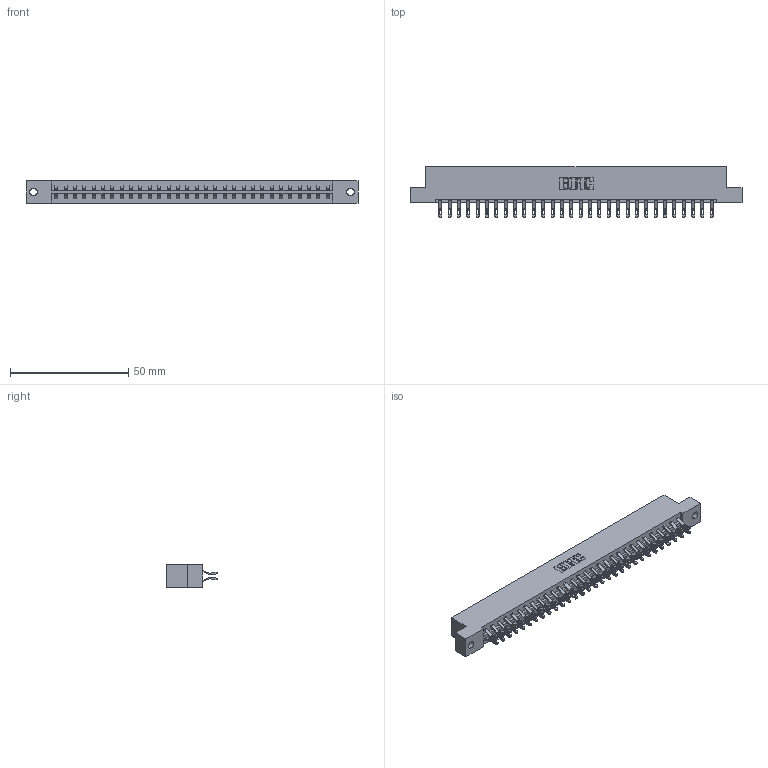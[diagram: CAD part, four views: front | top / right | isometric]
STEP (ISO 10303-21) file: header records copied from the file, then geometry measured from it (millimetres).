
FILE_DESCRIPTION (( 'STEP AP203' ), '1' );
FILE_NAME ('333-060-555-202.STEP', '2018-08-04T07:30:59', ( '' ), ( '' ), 'SwSTEP 2.0', 'SolidWorks 2016', '' );
FILE_SCHEMA (( 'CONFIG_CONTROL_DESIGN' ));
Length unit declared in the file: inch
Products named in the file (3): 333-060-555-202; 333 Part_Flush - .128 Dia; 345-292-001_555 Tail
Assembly tree (61 placements, depth 2):
  333-060-555-202
    333 Part_Flush - .128 Dia
    345-292-001_555 Tail  x60
Bounding box: 140.41 x 21.47 x 9.4 mm (x, y, z)
Volume: 14360.3 mm3; surface area: 17226 mm2
Topology: 61 solids, 61 shells, 3594 faces, 11291 edges, 7526 vertices
Faces by surface type: plane 2110, cylinder 1484
Entity records: 21181 total; most frequent: CARTESIAN_POINT 3560, ORIENTED_EDGE 3466, DIRECTION 3033, EDGE_CURVE 1733, LINE 1585, VECTOR 1585, VERTEX_POINT 1154, AXIS2_PLACEMENT_3D 724
